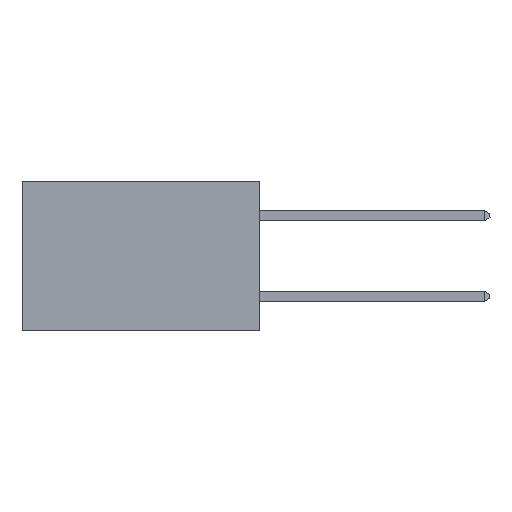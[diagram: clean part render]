
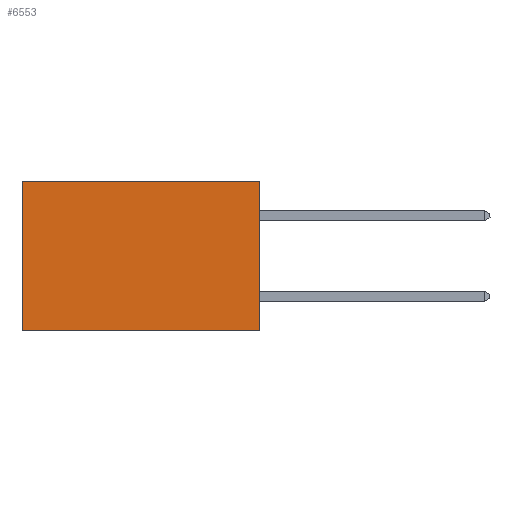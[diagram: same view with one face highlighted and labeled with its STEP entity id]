
A CAD part, left-side view. The second image highlights one B-rep face of the part: STEP entity #6553.
In plain terms, the highlighted planar face has unit normal (-1, 0, 0).
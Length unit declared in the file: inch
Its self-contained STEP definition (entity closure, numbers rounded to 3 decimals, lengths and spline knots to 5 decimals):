
#385 = CARTESIAN_POINT ( 'NONE',  ( 0.277, 0., -0.37 ) ) ;
#489 = EDGE_CURVE ( 'NONE', #1781, #4249, #6618, .T. ) ;
#852 = CARTESIAN_POINT ( 'NONE',  ( 0.277, 0., 0. ) ) ;
#1416 = ORIENTED_EDGE ( 'NONE', *, *, #7224, .F. ) ;
#1545 = CARTESIAN_POINT ( 'NONE',  ( 0.277, 0.59, -0.37 ) ) ;
#1652 = DIRECTION ( 'NONE',  ( 0., 0., -1. ) ) ;
#1781 = VERTEX_POINT ( 'NONE', #852 ) ;
#2203 = VECTOR ( 'NONE', #8520, 39.37008 ) ;
#2656 = VERTEX_POINT ( 'NONE', #4273 ) ;
#3104 = EDGE_LOOP ( 'NONE', ( #7413, #1416, #7226, #8509 ) ) ;
#3146 = FACE_OUTER_BOUND ( 'NONE', #3104, .T. ) ;
#3182 = VECTOR ( 'NONE', #6150, 39.37008 ) ;
#3621 = VERTEX_POINT ( 'NONE', #8451 ) ;
#3769 = CARTESIAN_POINT ( 'NONE',  ( 0.277, 0., -0.37 ) ) ;
#3942 = DIRECTION ( 'NONE',  ( 0., 1., 0. ) ) ;
#4249 = VERTEX_POINT ( 'NONE', #5195 ) ;
#4273 = CARTESIAN_POINT ( 'NONE',  ( 0.277, 0., -0.37 ) ) ;
#4430 = VECTOR ( 'NONE', #1652, 39.37008 ) ;
#5195 = CARTESIAN_POINT ( 'NONE',  ( 0.277, 0.59, 0. ) ) ;
#5435 = EDGE_CURVE ( 'NONE', #4249, #3621, #7830, .T. ) ;
#5536 = EDGE_CURVE ( 'NONE', #1781, #2656, #7208, .T. ) ;
#5646 = PLANE ( 'NONE',  #6349 ) ;
#5655 = CARTESIAN_POINT ( 'NONE',  ( 0.277, 0., -0.37 ) ) ;
#6150 = DIRECTION ( 'NONE',  ( 0., 1., 0. ) ) ;
#6349 = AXIS2_PLACEMENT_3D ( 'NONE', #5655, #7557, #7419 ) ;
#6553 = ADVANCED_FACE ( 'NONE', ( #3146 ), #5646, .F. ) ;
#6584 = VECTOR ( 'NONE', #3942, 39.37008 ) ;
#6618 = LINE ( 'NONE', #7663, #3182 ) ;
#7208 = LINE ( 'NONE', #385, #2203 ) ;
#7224 = EDGE_CURVE ( 'NONE', #2656, #3621, #8325, .T. ) ;
#7226 = ORIENTED_EDGE ( 'NONE', *, *, #5536, .F. ) ;
#7413 = ORIENTED_EDGE ( 'NONE', *, *, #5435, .T. ) ;
#7419 = DIRECTION ( 'NONE',  ( 0., 0., -1. ) ) ;
#7557 = DIRECTION ( 'NONE',  ( 1., 0., 0. ) ) ;
#7663 = CARTESIAN_POINT ( 'NONE',  ( 0.277, 0., 0. ) ) ;
#7830 = LINE ( 'NONE', #1545, #4430 ) ;
#8325 = LINE ( 'NONE', #3769, #6584 ) ;
#8451 = CARTESIAN_POINT ( 'NONE',  ( 0.277, 0.59, -0.37 ) ) ;
#8509 = ORIENTED_EDGE ( 'NONE', *, *, #489, .T. ) ;
#8520 = DIRECTION ( 'NONE',  ( 0., 0., -1. ) ) ;
